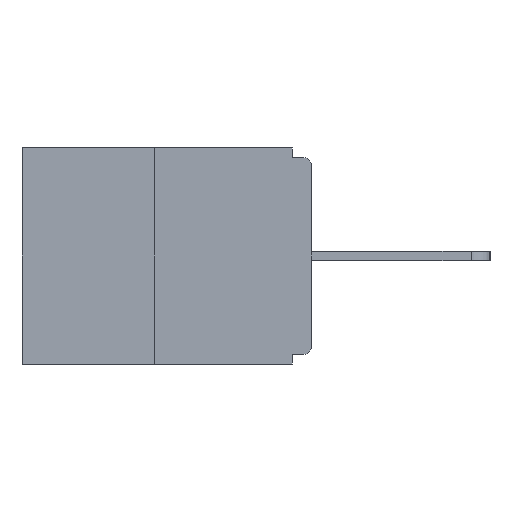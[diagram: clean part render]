
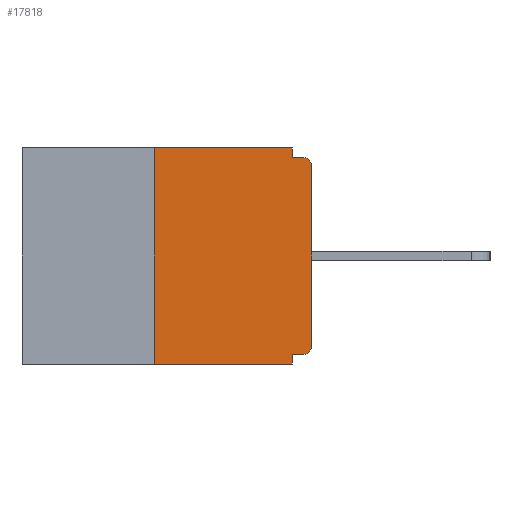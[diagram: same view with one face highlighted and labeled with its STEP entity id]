
A CAD part, left-side view. The second image highlights one B-rep face of the part: STEP entity #17818.
In plain terms, the highlighted planar face has unit normal (-1, 0, 0).
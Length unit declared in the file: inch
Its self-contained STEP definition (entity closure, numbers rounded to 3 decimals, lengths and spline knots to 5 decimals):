
#45 = VECTOR ( 'NONE', #8266, 39.37008 ) ;
#874 = EDGE_CURVE ( 'NONE', #11265, #5346, #18556, .T. ) ;
#1137 = DIRECTION ( 'NONE',  ( 0., 0., -1. ) ) ;
#1526 = VERTEX_POINT ( 'NONE', #20011 ) ;
#1619 = CARTESIAN_POINT ( 'NONE',  ( 0., 0., -0.03 ) ) ;
#2625 = CARTESIAN_POINT ( 'NONE',  ( 0., 0., -0.328 ) ) ;
#3216 = VERTEX_POINT ( 'NONE', #3608 ) ;
#3431 = CARTESIAN_POINT ( 'NONE',  ( 0., 0.25, 0. ) ) ;
#3608 = CARTESIAN_POINT ( 'NONE',  ( 0., 0.031, -0.328 ) ) ;
#4081 = EDGE_CURVE ( 'NONE', #21395, #14358, #7275, .T. ) ;
#4469 = EDGE_CURVE ( 'NONE', #6985, #13570, #23190, .T. ) ;
#4495 = DIRECTION ( 'NONE',  ( 1., 0., 0. ) ) ;
#5287 = EDGE_CURVE ( 'NONE', #3216, #14358, #23258, .T. ) ;
#5346 = VERTEX_POINT ( 'NONE', #9579 ) ;
#5607 = LINE ( 'NONE', #13522, #10602 ) ;
#5663 = CARTESIAN_POINT ( 'NONE',  ( 0., 0., 0. ) ) ;
#6171 = ORIENTED_EDGE ( 'NONE', *, *, #16209, .F. ) ;
#6631 = LINE ( 'NONE', #9070, #21547 ) ;
#6682 = DIRECTION ( 'NONE',  ( 0., 0., -1. ) ) ;
#6941 = EDGE_CURVE ( 'NONE', #17395, #6985, #10569, .T. ) ;
#6985 = VERTEX_POINT ( 'NONE', #7680 ) ;
#7071 = DIRECTION ( 'NONE',  ( -1., 0., 0. ) ) ;
#7275 = LINE ( 'NONE', #9573, #20322 ) ;
#7680 = CARTESIAN_POINT ( 'NONE',  ( 0., 0., -0.313 ) ) ;
#7793 = DIRECTION ( 'NONE',  ( 0., -1., 0. ) ) ;
#7914 = DIRECTION ( 'NONE',  ( 0., 0., -1. ) ) ;
#8003 = LINE ( 'NONE', #10307, #45 ) ;
#8266 = DIRECTION ( 'NONE',  ( 0., -1., 0. ) ) ;
#8957 = ORIENTED_EDGE ( 'NONE', *, *, #24780, .F. ) ;
#9070 = CARTESIAN_POINT ( 'NONE',  ( 0., 0.25, 0. ) ) ;
#9086 = EDGE_CURVE ( 'NONE', #21395, #24200, #6631, .T. ) ;
#9458 = DIRECTION ( 'NONE',  ( 0., -1., 0. ) ) ;
#9573 = CARTESIAN_POINT ( 'NONE',  ( 0., 0.46, -0.343 ) ) ;
#9579 = CARTESIAN_POINT ( 'NONE',  ( 0., 0.031, -0.015 ) ) ;
#10205 = AXIS2_PLACEMENT_3D ( 'NONE', #20489, #4495, #18170 ) ;
#10307 = CARTESIAN_POINT ( 'NONE',  ( 0., 0., -0.015 ) ) ;
#10569 = CIRCLE ( 'NONE', #24863, 0.015 ) ;
#10602 = VECTOR ( 'NONE', #7793, 39.37008 ) ;
#10624 = CARTESIAN_POINT ( 'NONE',  ( 0., 0.031, 0. ) ) ;
#10671 = ORIENTED_EDGE ( 'NONE', *, *, #4081, .T. ) ;
#11146 = CARTESIAN_POINT ( 'NONE',  ( 0., 0.031, -0.343 ) ) ;
#11265 = VERTEX_POINT ( 'NONE', #21696 ) ;
#11733 = CARTESIAN_POINT ( 'NONE',  ( 0., 0.031, -0.343 ) ) ;
#11832 = EDGE_LOOP ( 'NONE', ( #6171, #13688, #10671, #16300, #22200, #13024, #25275, #18601, #8957, #23636 ) ) ;
#11961 = DIRECTION ( 'NONE',  ( 0., 0., -1. ) ) ;
#13024 = ORIENTED_EDGE ( 'NONE', *, *, #6941, .T. ) ;
#13522 = CARTESIAN_POINT ( 'NONE',  ( 0., 0.46, 0. ) ) ;
#13570 = VERTEX_POINT ( 'NONE', #1619 ) ;
#13688 = ORIENTED_EDGE ( 'NONE', *, *, #9086, .F. ) ;
#14358 = VERTEX_POINT ( 'NONE', #11146 ) ;
#14406 = VECTOR ( 'NONE', #1137, 39.37008 ) ;
#14564 = FACE_OUTER_BOUND ( 'NONE', #11832, .T. ) ;
#14958 = VECTOR ( 'NONE', #23326, 39.37008 ) ;
#15776 = CARTESIAN_POINT ( 'NONE',  ( 0., 0.015, -0.03 ) ) ;
#16209 = EDGE_CURVE ( 'NONE', #24200, #11265, #5607, .T. ) ;
#16300 = ORIENTED_EDGE ( 'NONE', *, *, #5287, .F. ) ;
#17395 = VERTEX_POINT ( 'NONE', #24335 ) ;
#17818 = ADVANCED_FACE ( 'NONE', ( #14564 ), #24186, .F. ) ;
#18170 = DIRECTION ( 'NONE',  ( 0., 0., -1. ) ) ;
#18556 = LINE ( 'NONE', #10624, #14406 ) ;
#18601 = ORIENTED_EDGE ( 'NONE', *, *, #19041, .T. ) ;
#19041 = EDGE_CURVE ( 'NONE', #13570, #1526, #21296, .T. ) ;
#19557 = CARTESIAN_POINT ( 'NONE',  ( 0., 0.25, -0.343 ) ) ;
#20011 = CARTESIAN_POINT ( 'NONE',  ( 0., 0.015, -0.015 ) ) ;
#20037 = VECTOR ( 'NONE', #24135, 39.37008 ) ;
#20322 = VECTOR ( 'NONE', #9458, 39.37008 ) ;
#20489 = CARTESIAN_POINT ( 'NONE',  ( 0., 0.46, 0. ) ) ;
#20503 = CARTESIAN_POINT ( 'NONE',  ( 0., 0.015, -0.313 ) ) ;
#21296 = CIRCLE ( 'NONE', #21706, 0.015 ) ;
#21395 = VERTEX_POINT ( 'NONE', #19557 ) ;
#21547 = VECTOR ( 'NONE', #22628, 39.37008 ) ;
#21696 = CARTESIAN_POINT ( 'NONE',  ( 0., 0.031, 0. ) ) ;
#21702 = DIRECTION ( 'NONE',  ( -1., 0., 0. ) ) ;
#21706 = AXIS2_PLACEMENT_3D ( 'NONE', #15776, #21702, #11961 ) ;
#22200 = ORIENTED_EDGE ( 'NONE', *, *, #23241, .F. ) ;
#22628 = DIRECTION ( 'NONE',  ( 0., 0., 1. ) ) ;
#23190 = LINE ( 'NONE', #5663, #14958 ) ;
#23241 = EDGE_CURVE ( 'NONE', #17395, #3216, #24002, .T. ) ;
#23258 = LINE ( 'NONE', #11733, #23593 ) ;
#23326 = DIRECTION ( 'NONE',  ( 0., 0., 1. ) ) ;
#23593 = VECTOR ( 'NONE', #7914, 39.37008 ) ;
#23636 = ORIENTED_EDGE ( 'NONE', *, *, #874, .F. ) ;
#24002 = LINE ( 'NONE', #2625, #20037 ) ;
#24135 = DIRECTION ( 'NONE',  ( 0., 1., 0. ) ) ;
#24186 = PLANE ( 'NONE',  #10205 ) ;
#24200 = VERTEX_POINT ( 'NONE', #3431 ) ;
#24335 = CARTESIAN_POINT ( 'NONE',  ( 0., 0.015, -0.328 ) ) ;
#24780 = EDGE_CURVE ( 'NONE', #5346, #1526, #8003, .T. ) ;
#24863 = AXIS2_PLACEMENT_3D ( 'NONE', #20503, #7071, #6682 ) ;
#25275 = ORIENTED_EDGE ( 'NONE', *, *, #4469, .T. ) ;
